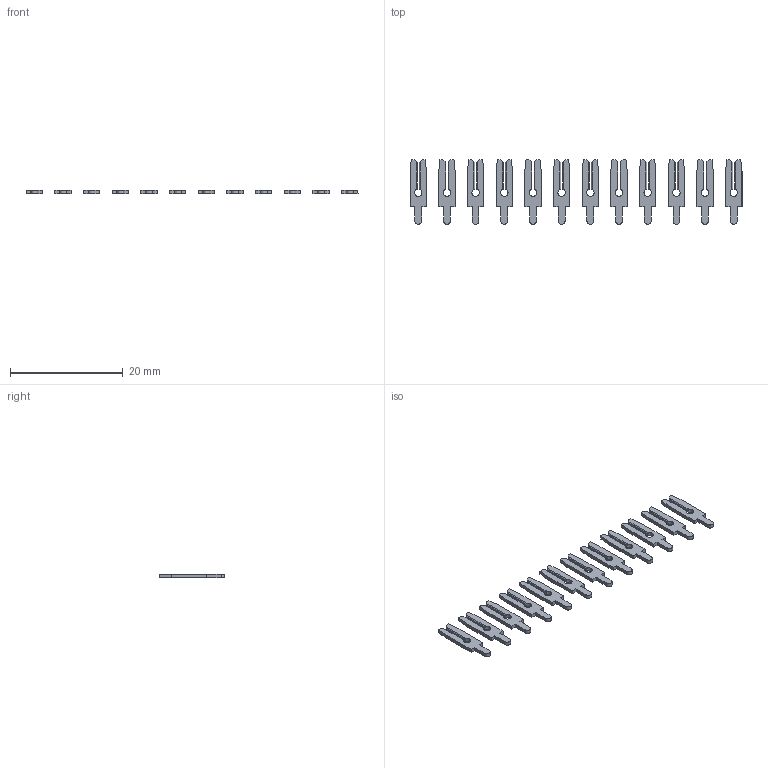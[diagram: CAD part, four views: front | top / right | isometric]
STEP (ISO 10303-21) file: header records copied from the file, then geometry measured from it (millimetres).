
FILE_DESCRIPTION (( 'STEP AP203' ), '1' );
FILE_NAME ('103-012-250-200.STEP', '2020-04-09T19:49:45', ( '' ), ( '' ), 'SwSTEP 2.0', 'SolidWorks 2016', '' );
FILE_SCHEMA (( 'CONFIG_CONTROL_DESIGN' ));
Length unit declared in the file: inch
Products named in the file (2): 100-290-001_100-290-250; 103-012-250-200
Assembly tree (12 placements, depth 2):
  103-012-250-200
    100-290-001_100-290-250  x12
Bounding box: 58.8 x 11.48 x 0.66 mm (x, y, z)
Volume: 187.3 mm3; surface area: 880.2 mm2
Topology: 12 solids, 12 shells, 288 faces, 792 edges, 528 vertices
Faces by surface type: plane 240, cylinder 48
Entity records: 1310 total; most frequent: CARTESIAN_POINT 161, DIRECTION 148, ORIENTED_EDGE 132, EDGE_CURVE 66, VECTOR 54, LINE 54, AXIS2_PLACEMENT_3D 47, VERTEX_POINT 44
